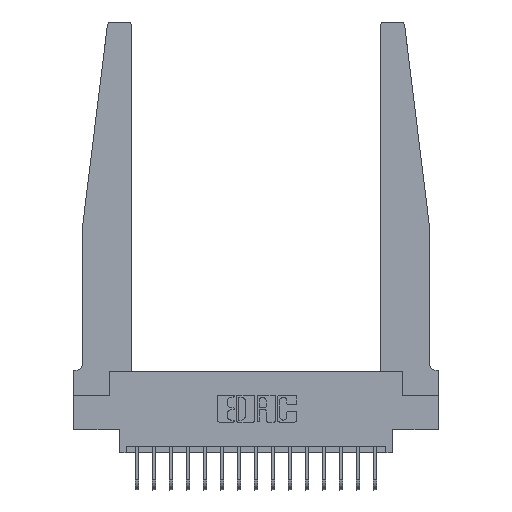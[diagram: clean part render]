
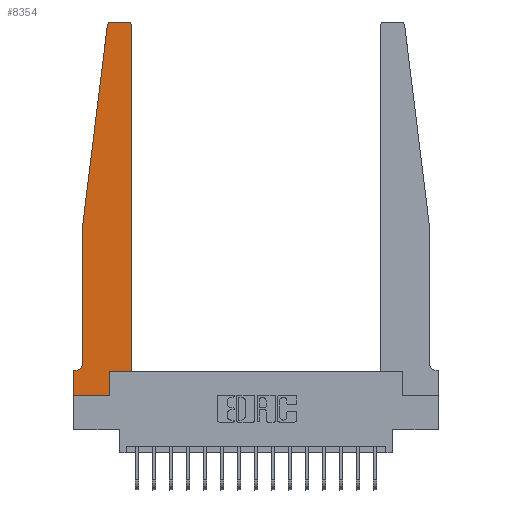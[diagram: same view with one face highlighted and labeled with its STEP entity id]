
A CAD part, top view. The second image highlights one B-rep face of the part: STEP entity #8354.
In plain terms, the highlighted planar face has unit normal (0, 0, 1).
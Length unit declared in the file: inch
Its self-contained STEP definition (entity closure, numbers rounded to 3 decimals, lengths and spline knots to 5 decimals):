
#200 = EDGE_CURVE ( 'NONE', #6074, #8566, #3426, .T. ) ;
#287 = DIRECTION ( 'NONE',  ( 0., 1., 0. ) ) ;
#357 = ORIENTED_EDGE ( 'NONE', *, *, #12633, .T. ) ;
#626 = CIRCLE ( 'NONE', #11477, 0.05 ) ;
#670 = CARTESIAN_POINT ( 'NONE',  ( 0., 0.1875, 0.37 ) ) ;
#786 = ORIENTED_EDGE ( 'NONE', *, *, #9952, .T. ) ;
#1000 = ORIENTED_EDGE ( 'NONE', *, *, #3454, .T. ) ;
#1082 = CARTESIAN_POINT ( 'NONE',  ( 0.395, 2.72, 0.37 ) ) ;
#1098 = DIRECTION ( 'NONE',  ( -1., 0., 0. ) ) ;
#1126 = CARTESIAN_POINT ( 'NONE',  ( 0.015, 0.1875, 0.37 ) ) ;
#1147 = VERTEX_POINT ( 'NONE', #7976 ) ;
#1449 = VECTOR ( 'NONE', #4480, 39.37008 ) ;
#1485 = EDGE_CURVE ( 'NONE', #8566, #8647, #2214, .T. ) ;
#1573 = CARTESIAN_POINT ( 'NONE',  ( 0.25, 2.75, 0.37 ) ) ;
#1707 = LINE ( 'NONE', #7354, #16046 ) ;
#2214 = CIRCLE ( 'NONE', #6064, 0.03 ) ;
#2455 = EDGE_CURVE ( 'NONE', #13868, #5094, #626, .T. ) ;
#2518 = DIRECTION ( 'NONE',  ( 1., 0., 0. ) ) ;
#3426 = LINE ( 'NONE', #12671, #8007 ) ;
#3442 = DIRECTION ( 'NONE',  ( 0., -1., 0. ) ) ;
#3454 = EDGE_CURVE ( 'NONE', #5289, #6582, #17483, .T. ) ;
#4039 = EDGE_CURVE ( 'NONE', #10819, #6074, #8483, .T. ) ;
#4112 = VECTOR ( 'NONE', #13139, 39.37008 ) ;
#4461 = VERTEX_POINT ( 'NONE', #670 ) ;
#4480 = DIRECTION ( 'NONE',  ( -1., 0., 0. ) ) ;
#4635 = CARTESIAN_POINT ( 'NONE',  ( 0.24675, 2.72367, 0.37 ) ) ;
#5039 = ORIENTED_EDGE ( 'NONE', *, *, #9739, .T. ) ;
#5094 = VERTEX_POINT ( 'NONE', #1126 ) ;
#5128 = CARTESIAN_POINT ( 'NONE',  ( 0.065, 0.1875, 0.37 ) ) ;
#5270 = LINE ( 'NONE', #1573, #1449 ) ;
#5289 = VERTEX_POINT ( 'NONE', #10023 ) ;
#6064 = AXIS2_PLACEMENT_3D ( 'NONE', #1082, #10896, #2518 ) ;
#6074 = VERTEX_POINT ( 'NONE', #10549 ) ;
#6582 = VERTEX_POINT ( 'NONE', #4635 ) ;
#6595 = CARTESIAN_POINT ( 'NONE',  ( 0.395, 2.75, 0.37 ) ) ;
#6824 = CARTESIAN_POINT ( 'NONE',  ( 0.425, 0.18, 0.37 ) ) ;
#6830 = CARTESIAN_POINT ( 'NONE',  ( 0.27653, 2.72, 0.37 ) ) ;
#6973 = LINE ( 'NONE', #5128, #17859 ) ;
#7088 = DIRECTION ( 'NONE',  ( 0., 0., 1. ) ) ;
#7354 = CARTESIAN_POINT ( 'NONE',  ( 0.2605, 0.18, 0.37 ) ) ;
#7473 = CARTESIAN_POINT ( 'NONE',  ( 0.065, 1.25, 0.37 ) ) ;
#7516 = VERTEX_POINT ( 'NONE', #16313 ) ;
#7696 = CARTESIAN_POINT ( 'NONE',  ( 0.425, 2.72, 0.37 ) ) ;
#7788 = EDGE_CURVE ( 'NONE', #7516, #10819, #1707, .T. ) ;
#7871 = DIRECTION ( 'NONE',  ( -1., 0., 0. ) ) ;
#7976 = CARTESIAN_POINT ( 'NONE',  ( 0., 0., 0.37 ) ) ;
#8000 = DIRECTION ( 'NONE',  ( -0.122, -0.992, 0. ) ) ;
#8007 = VECTOR ( 'NONE', #13337, 39.37008 ) ;
#8212 = DIRECTION ( 'NONE',  ( 1., 0., 0. ) ) ;
#8219 = DIRECTION ( 'NONE',  ( 1., 0., 0. ) ) ;
#8296 = ORIENTED_EDGE ( 'NONE', *, *, #2455, .T. ) ;
#8354 = ADVANCED_FACE ( 'NONE', ( #15187 ), #13943, .T. ) ;
#8483 = LINE ( 'NONE', #6824, #11733 ) ;
#8566 = VERTEX_POINT ( 'NONE', #7696 ) ;
#8644 = VECTOR ( 'NONE', #8000, 39.37008 ) ;
#8647 = VERTEX_POINT ( 'NONE', #6595 ) ;
#8835 = DIRECTION ( 'NONE',  ( 0., -1., 0. ) ) ;
#9498 = DIRECTION ( 'NONE',  ( 0., 0., -1. ) ) ;
#9739 = EDGE_CURVE ( 'NONE', #14800, #13868, #10424, .T. ) ;
#9952 = EDGE_CURVE ( 'NONE', #5094, #4461, #6973, .T. ) ;
#10023 = CARTESIAN_POINT ( 'NONE',  ( 0.27653, 2.75, 0.37 ) ) ;
#10415 = CARTESIAN_POINT ( 'NONE',  ( 0., 0., 0.37 ) ) ;
#10424 = LINE ( 'NONE', #7473, #17657 ) ;
#10549 = CARTESIAN_POINT ( 'NONE',  ( 0.425, 0.18, 0.37 ) ) ;
#10657 = ORIENTED_EDGE ( 'NONE', *, *, #4039, .T. ) ;
#10819 = VERTEX_POINT ( 'NONE', #15153 ) ;
#10896 = DIRECTION ( 'NONE',  ( 0., 0., 1. ) ) ;
#11096 = ORIENTED_EDGE ( 'NONE', *, *, #17081, .T. ) ;
#11367 = EDGE_CURVE ( 'NONE', #6582, #14800, #15929, .T. ) ;
#11477 = AXIS2_PLACEMENT_3D ( 'NONE', #17669, #9498, #1098 ) ;
#11708 = CARTESIAN_POINT ( 'NONE',  ( 0.065, 0.2375, 0.37 ) ) ;
#11733 = VECTOR ( 'NONE', #8212, 39.37008 ) ;
#12175 = ORIENTED_EDGE ( 'NONE', *, *, #15609, .T. ) ;
#12404 = ORIENTED_EDGE ( 'NONE', *, *, #11367, .T. ) ;
#12633 = EDGE_CURVE ( 'NONE', #4461, #1147, #16079, .T. ) ;
#12671 = CARTESIAN_POINT ( 'NONE',  ( 0.425, 0.18, 0.37 ) ) ;
#12904 = VECTOR ( 'NONE', #3442, 39.37008 ) ;
#13139 = DIRECTION ( 'NONE',  ( 1., 0., 0. ) ) ;
#13337 = DIRECTION ( 'NONE',  ( 0., 1., 0. ) ) ;
#13868 = VERTEX_POINT ( 'NONE', #11708 ) ;
#13943 = PLANE ( 'NONE',  #16309 ) ;
#14337 = ORIENTED_EDGE ( 'NONE', *, *, #7788, .T. ) ;
#14800 = VERTEX_POINT ( 'NONE', #16405 ) ;
#14993 = EDGE_LOOP ( 'NONE', ( #12175, #1000, #12404, #5039, #8296, #786, #357, #11096, #14337, #10657, #16832, #16407 ) ) ;
#15153 = CARTESIAN_POINT ( 'NONE',  ( 0.2605, 0.18, 0.37 ) ) ;
#15187 = FACE_OUTER_BOUND ( 'NONE', #14993, .T. ) ;
#15295 = CARTESIAN_POINT ( 'NONE',  ( 0., 0.1875, 0.37 ) ) ;
#15609 = EDGE_CURVE ( 'NONE', #8647, #5289, #5270, .T. ) ;
#15929 = LINE ( 'NONE', #16178, #8644 ) ;
#15933 = AXIS2_PLACEMENT_3D ( 'NONE', #6830, #16397, #8219 ) ;
#16046 = VECTOR ( 'NONE', #287, 39.37008 ) ;
#16079 = LINE ( 'NONE', #10415, #12904 ) ;
#16178 = CARTESIAN_POINT ( 'NONE',  ( 0.065, 1.25, 0.37 ) ) ;
#16309 = AXIS2_PLACEMENT_3D ( 'NONE', #15295, #7088, #16637 ) ;
#16313 = CARTESIAN_POINT ( 'NONE',  ( 0.2605, 0., 0.37 ) ) ;
#16397 = DIRECTION ( 'NONE',  ( 0., 0., 1. ) ) ;
#16405 = CARTESIAN_POINT ( 'NONE',  ( 0.065, 1.25, 0.37 ) ) ;
#16407 = ORIENTED_EDGE ( 'NONE', *, *, #1485, .T. ) ;
#16637 = DIRECTION ( 'NONE',  ( 1., 0., 0. ) ) ;
#16832 = ORIENTED_EDGE ( 'NONE', *, *, #200, .T. ) ;
#17081 = EDGE_CURVE ( 'NONE', #1147, #7516, #17849, .T. ) ;
#17229 = CARTESIAN_POINT ( 'NONE',  ( 0., 0., 0.37 ) ) ;
#17483 = CIRCLE ( 'NONE', #15933, 0.03 ) ;
#17657 = VECTOR ( 'NONE', #8835, 39.37008 ) ;
#17669 = CARTESIAN_POINT ( 'NONE',  ( 0.015, 0.2375, 0.37 ) ) ;
#17849 = LINE ( 'NONE', #17229, #4112 ) ;
#17859 = VECTOR ( 'NONE', #7871, 39.37008 ) ;
